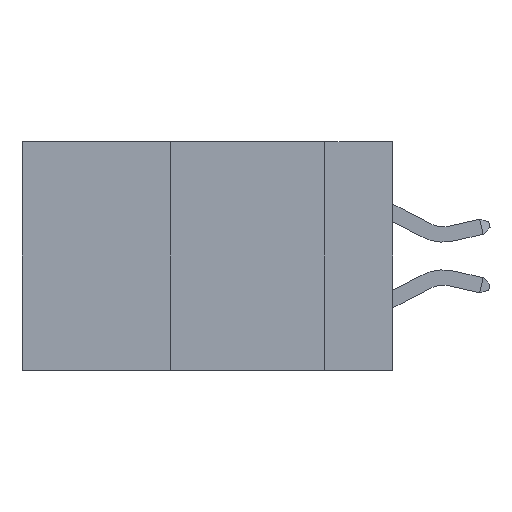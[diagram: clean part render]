
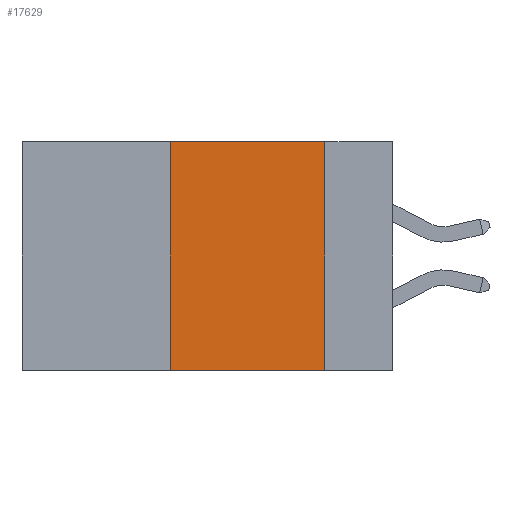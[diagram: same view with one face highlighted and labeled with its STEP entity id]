
A CAD part, left-side view. The second image highlights one B-rep face of the part: STEP entity #17629.
In plain terms, the highlighted planar face has unit normal (-1, 0, 0).
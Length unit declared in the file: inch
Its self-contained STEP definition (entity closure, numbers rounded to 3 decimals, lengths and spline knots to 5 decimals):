
#1118 = ORIENTED_EDGE ( 'NONE', *, *, #21971, .F. ) ;
#1279 = CARTESIAN_POINT ( 'NONE',  ( 0., 0.11, -0.37 ) ) ;
#1432 = VERTEX_POINT ( 'NONE', #15326 ) ;
#2641 = ORIENTED_EDGE ( 'NONE', *, *, #13840, .F. ) ;
#4796 = VERTEX_POINT ( 'NONE', #18525 ) ;
#5331 = VECTOR ( 'NONE', #11811, 39.37008 ) ;
#6094 = ORIENTED_EDGE ( 'NONE', *, *, #10877, .T. ) ;
#7492 = FACE_OUTER_BOUND ( 'NONE', #8886, .T. ) ;
#7551 = PLANE ( 'NONE',  #10992 ) ;
#8886 = EDGE_LOOP ( 'NONE', ( #18092, #1118, #2641, #6094 ) ) ;
#9082 = LINE ( 'NONE', #11681, #12687 ) ;
#10222 = DIRECTION ( 'NONE',  ( 0., 0., -1. ) ) ;
#10877 = EDGE_CURVE ( 'NONE', #4796, #19572, #14773, .T. ) ;
#10992 = AXIS2_PLACEMENT_3D ( 'NONE', #19681, #18049, #12748 ) ;
#11681 = CARTESIAN_POINT ( 'NONE',  ( 0., 0.11, 0. ) ) ;
#11811 = DIRECTION ( 'NONE',  ( 0., -1., 0. ) ) ;
#12114 = VERTEX_POINT ( 'NONE', #16015 ) ;
#12687 = VECTOR ( 'NONE', #10222, 39.37008 ) ;
#12748 = DIRECTION ( 'NONE',  ( 0., 0., -1. ) ) ;
#13840 = EDGE_CURVE ( 'NONE', #4796, #1432, #15193, .T. ) ;
#14592 = VECTOR ( 'NONE', #22150, 39.37008 ) ;
#14773 = LINE ( 'NONE', #21935, #5331 ) ;
#15193 = LINE ( 'NONE', #17088, #22931 ) ;
#15225 = DIRECTION ( 'NONE',  ( 0., 0., 1. ) ) ;
#15326 = CARTESIAN_POINT ( 'NONE',  ( 0., 0.36, 0. ) ) ;
#16015 = CARTESIAN_POINT ( 'NONE',  ( 0., 0.11, 0. ) ) ;
#17088 = CARTESIAN_POINT ( 'NONE',  ( 0., 0.36, 0. ) ) ;
#17629 = ADVANCED_FACE ( 'NONE', ( #7492 ), #7551, .F. ) ;
#18049 = DIRECTION ( 'NONE',  ( 1., 0., 0. ) ) ;
#18092 = ORIENTED_EDGE ( 'NONE', *, *, #19559, .F. ) ;
#18525 = CARTESIAN_POINT ( 'NONE',  ( 0., 0.36, -0.37 ) ) ;
#18673 = CARTESIAN_POINT ( 'NONE',  ( 0., 0.6, 0. ) ) ;
#19559 = EDGE_CURVE ( 'NONE', #12114, #19572, #9082, .T. ) ;
#19572 = VERTEX_POINT ( 'NONE', #1279 ) ;
#19681 = CARTESIAN_POINT ( 'NONE',  ( 0., 0.6, 0. ) ) ;
#21827 = LINE ( 'NONE', #18673, #14592 ) ;
#21935 = CARTESIAN_POINT ( 'NONE',  ( 0., 0.6, -0.37 ) ) ;
#21971 = EDGE_CURVE ( 'NONE', #1432, #12114, #21827, .T. ) ;
#22150 = DIRECTION ( 'NONE',  ( 0., -1., 0. ) ) ;
#22931 = VECTOR ( 'NONE', #15225, 39.37008 ) ;
